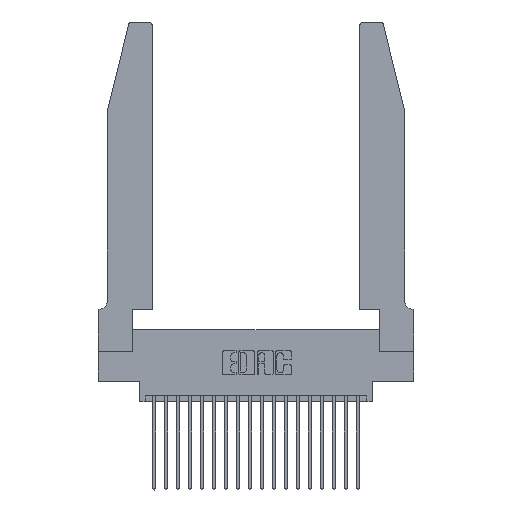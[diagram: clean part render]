
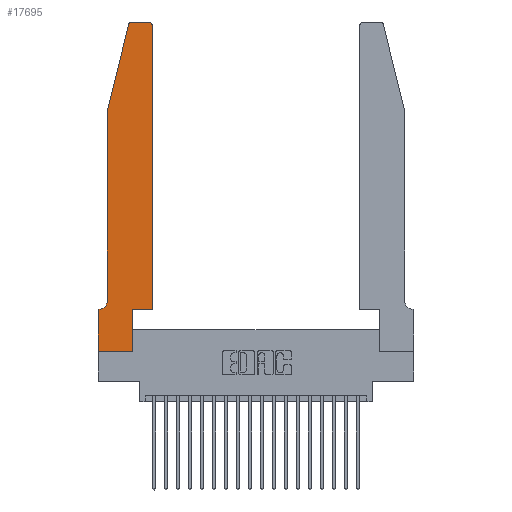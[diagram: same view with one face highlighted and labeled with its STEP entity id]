
A CAD part, top view. The second image highlights one B-rep face of the part: STEP entity #17695.
In plain terms, the highlighted planar face has unit normal (0, 0, 1).
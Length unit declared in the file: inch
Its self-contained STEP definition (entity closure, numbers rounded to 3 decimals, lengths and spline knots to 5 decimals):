
#177 = EDGE_CURVE ( 'NONE', #17470, #10919, #4652, .T. ) ;
#363 = VECTOR ( 'NONE', #16721, 39.37008 ) ;
#716 = ORIENTED_EDGE ( 'NONE', *, *, #21187, .T. ) ;
#1029 = CARTESIAN_POINT ( 'NONE',  ( 0.284, 2.72, 0.37 ) ) ;
#1148 = DIRECTION ( 'NONE',  ( 1., 0., 0. ) ) ;
#1250 = VECTOR ( 'NONE', #7567, 39.37008 ) ;
#1512 = CIRCLE ( 'NONE', #8789, 0.03 ) ;
#1611 = VERTEX_POINT ( 'NONE', #5097 ) ;
#1693 = CARTESIAN_POINT ( 'NONE',  ( 0.4205, 2.72, 0.37 ) ) ;
#1848 = ORIENTED_EDGE ( 'NONE', *, *, #18274, .T. ) ;
#1942 = EDGE_CURVE ( 'NONE', #1611, #17470, #12437, .T. ) ;
#1980 = VERTEX_POINT ( 'NONE', #13576 ) ;
#2391 = DIRECTION ( 'NONE',  ( -0.239, -0.971, 0. ) ) ;
#3020 = VERTEX_POINT ( 'NONE', #15649 ) ;
#3132 = EDGE_CURVE ( 'NONE', #9112, #6432, #10383, .T. ) ;
#3298 = DIRECTION ( 'NONE',  ( -1., 0., 0. ) ) ;
#3416 = VERTEX_POINT ( 'NONE', #19211 ) ;
#3436 = ORIENTED_EDGE ( 'NONE', *, *, #7310, .T. ) ;
#3468 = CARTESIAN_POINT ( 'NONE',  ( 0., 0., 0.37 ) ) ;
#3523 = AXIS2_PLACEMENT_3D ( 'NONE', #13234, #18360, #1148 ) ;
#3549 = VERTEX_POINT ( 'NONE', #8555 ) ;
#3711 = EDGE_CURVE ( 'NONE', #21509, #3020, #19208, .T. ) ;
#4011 = EDGE_CURVE ( 'NONE', #1980, #6386, #8145, .T. ) ;
#4592 = LINE ( 'NONE', #22055, #9181 ) ;
#4652 = LINE ( 'NONE', #15102, #6539 ) ;
#4886 = LINE ( 'NONE', #3468, #18895 ) ;
#4887 = VECTOR ( 'NONE', #2391, 39.37008 ) ;
#4951 = DIRECTION ( 'NONE',  ( 0., 0., -1. ) ) ;
#5097 = CARTESIAN_POINT ( 'NONE',  ( 0.2865, 0., 0.37 ) ) ;
#5105 = CARTESIAN_POINT ( 'NONE',  ( 0.0055, 0.42, 0.37 ) ) ;
#5143 = CARTESIAN_POINT ( 'NONE',  ( 0.2865, 0.35, 0.37 ) ) ;
#5762 = VECTOR ( 'NONE', #21402, 39.37008 ) ;
#5781 = CARTESIAN_POINT ( 'NONE',  ( 0., 0.35, 0.37 ) ) ;
#5858 = AXIS2_PLACEMENT_3D ( 'NONE', #5105, #4951, #15596 ) ;
#5898 = CARTESIAN_POINT ( 'NONE',  ( 0.0755, 2., 0.37 ) ) ;
#6386 = VERTEX_POINT ( 'NONE', #7764 ) ;
#6432 = VERTEX_POINT ( 'NONE', #21307 ) ;
#6539 = VECTOR ( 'NONE', #8302, 39.37008 ) ;
#7310 = EDGE_CURVE ( 'NONE', #3416, #21509, #13184, .T. ) ;
#7546 = LINE ( 'NONE', #14520, #4887 ) ;
#7567 = DIRECTION ( 'NONE',  ( -1., 0., 0. ) ) ;
#7764 = CARTESIAN_POINT ( 'NONE',  ( 0.4205, 2.75, 0.37 ) ) ;
#7845 = CARTESIAN_POINT ( 'NONE',  ( 0.4505, 0.35, 0.37 ) ) ;
#8135 = DIRECTION ( 'NONE',  ( 0., 1., 0. ) ) ;
#8145 = CIRCLE ( 'NONE', #21359, 0.03 ) ;
#8240 = CARTESIAN_POINT ( 'NONE',  ( 0., 0., 0.37 ) ) ;
#8302 = DIRECTION ( 'NONE',  ( 1., 0., 0. ) ) ;
#8364 = EDGE_CURVE ( 'NONE', #15326, #3549, #1512, .T. ) ;
#8415 = CARTESIAN_POINT ( 'NONE',  ( 0.0755, 0.35, 0.37 ) ) ;
#8555 = CARTESIAN_POINT ( 'NONE',  ( 0.25487, 2.72718, 0.37 ) ) ;
#8608 = VECTOR ( 'NONE', #13441, 39.37008 ) ;
#8789 = AXIS2_PLACEMENT_3D ( 'NONE', #1029, #13108, #11274 ) ;
#9015 = EDGE_CURVE ( 'NONE', #6432, #3416, #16891, .T. ) ;
#9112 = VERTEX_POINT ( 'NONE', #9977 ) ;
#9181 = VECTOR ( 'NONE', #8135, 39.37008 ) ;
#9977 = CARTESIAN_POINT ( 'NONE',  ( 0.0755, 2., 0.37 ) ) ;
#10383 = LINE ( 'NONE', #5898, #5762 ) ;
#10412 = LINE ( 'NONE', #16352, #1250 ) ;
#10439 = FACE_OUTER_BOUND ( 'NONE', #14697, .T. ) ;
#10473 = EDGE_CURVE ( 'NONE', #3549, #9112, #7546, .T. ) ;
#10919 = VERTEX_POINT ( 'NONE', #7845 ) ;
#11274 = DIRECTION ( 'NONE',  ( 1., 0., 0. ) ) ;
#11883 = ORIENTED_EDGE ( 'NONE', *, *, #3711, .T. ) ;
#11905 = ORIENTED_EDGE ( 'NONE', *, *, #3132, .T. ) ;
#12051 = ORIENTED_EDGE ( 'NONE', *, *, #9015, .T. ) ;
#12437 = LINE ( 'NONE', #21946, #8608 ) ;
#12771 = ORIENTED_EDGE ( 'NONE', *, *, #1942, .T. ) ;
#12897 = CARTESIAN_POINT ( 'NONE',  ( 0.284, 2.75, 0.37 ) ) ;
#13108 = DIRECTION ( 'NONE',  ( 0., 0., 1. ) ) ;
#13169 = ORIENTED_EDGE ( 'NONE', *, *, #21294, .T. ) ;
#13184 = LINE ( 'NONE', #8415, #15315 ) ;
#13234 = CARTESIAN_POINT ( 'NONE',  ( 0., 0.35, 0.37 ) ) ;
#13441 = DIRECTION ( 'NONE',  ( 0., 1., 0. ) ) ;
#13576 = CARTESIAN_POINT ( 'NONE',  ( 0.4505, 2.72, 0.37 ) ) ;
#13695 = DIRECTION ( 'NONE',  ( 1., 0., 0. ) ) ;
#14520 = CARTESIAN_POINT ( 'NONE',  ( 0.0755, 2., 0.37 ) ) ;
#14697 = EDGE_LOOP ( 'NONE', ( #1848, #21132, #17572, #11905, #12051, #3436, #11883, #13169, #12771, #17591, #716, #20244 ) ) ;
#15102 = CARTESIAN_POINT ( 'NONE',  ( 0.4505, 0.35, 0.37 ) ) ;
#15315 = VECTOR ( 'NONE', #3298, 39.37008 ) ;
#15326 = VERTEX_POINT ( 'NONE', #12897 ) ;
#15333 = DIRECTION ( 'NONE',  ( 0., 0., 1. ) ) ;
#15596 = DIRECTION ( 'NONE',  ( -1., 0., 0. ) ) ;
#15649 = CARTESIAN_POINT ( 'NONE',  ( 0., 0., 0.37 ) ) ;
#15698 = DIRECTION ( 'NONE',  ( 1., 0., 0. ) ) ;
#16352 = CARTESIAN_POINT ( 'NONE',  ( 0.2605, 2.75, 0.37 ) ) ;
#16721 = DIRECTION ( 'NONE',  ( 0., -1., 0. ) ) ;
#16891 = CIRCLE ( 'NONE', #5858, 0.07 ) ;
#17470 = VERTEX_POINT ( 'NONE', #5143 ) ;
#17572 = ORIENTED_EDGE ( 'NONE', *, *, #10473, .T. ) ;
#17591 = ORIENTED_EDGE ( 'NONE', *, *, #177, .T. ) ;
#17695 = ADVANCED_FACE ( 'NONE', ( #10439 ), #21285, .T. ) ;
#18274 = EDGE_CURVE ( 'NONE', #6386, #15326, #10412, .T. ) ;
#18360 = DIRECTION ( 'NONE',  ( 0., 0., 1. ) ) ;
#18895 = VECTOR ( 'NONE', #15698, 39.37008 ) ;
#19208 = LINE ( 'NONE', #8240, #363 ) ;
#19211 = CARTESIAN_POINT ( 'NONE',  ( 0.0055, 0.35, 0.37 ) ) ;
#20244 = ORIENTED_EDGE ( 'NONE', *, *, #4011, .T. ) ;
#21132 = ORIENTED_EDGE ( 'NONE', *, *, #8364, .T. ) ;
#21187 = EDGE_CURVE ( 'NONE', #10919, #1980, #4592, .T. ) ;
#21285 = PLANE ( 'NONE',  #3523 ) ;
#21294 = EDGE_CURVE ( 'NONE', #3020, #1611, #4886, .T. ) ;
#21307 = CARTESIAN_POINT ( 'NONE',  ( 0.0755, 0.42, 0.37 ) ) ;
#21359 = AXIS2_PLACEMENT_3D ( 'NONE', #1693, #15333, #13695 ) ;
#21402 = DIRECTION ( 'NONE',  ( 0., -1., 0. ) ) ;
#21509 = VERTEX_POINT ( 'NONE', #5781 ) ;
#21946 = CARTESIAN_POINT ( 'NONE',  ( 0.2865, 0.35, 0.37 ) ) ;
#22055 = CARTESIAN_POINT ( 'NONE',  ( 0.4505, 0.35, 0.37 ) ) ;
